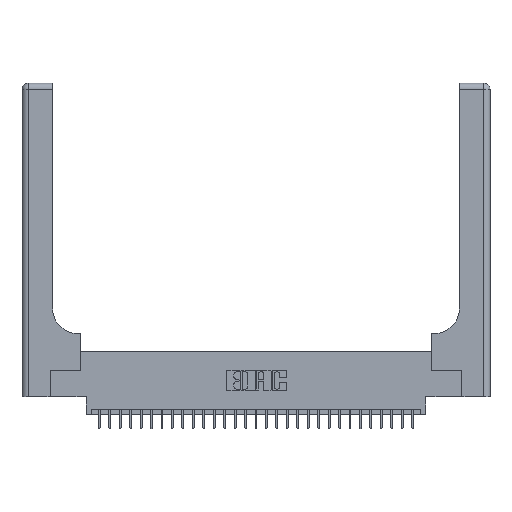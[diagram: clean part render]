
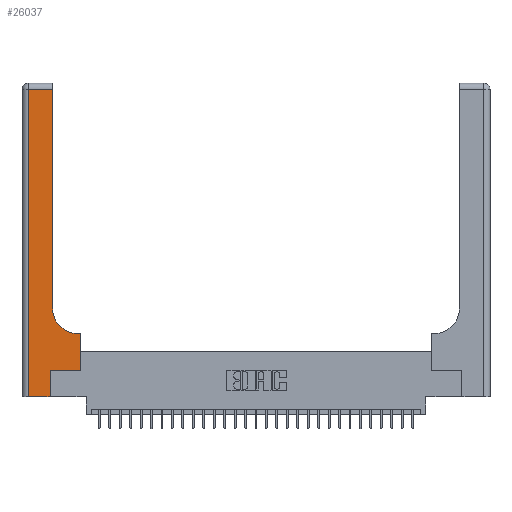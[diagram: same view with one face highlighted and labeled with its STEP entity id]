
A CAD part, top view. The second image highlights one B-rep face of the part: STEP entity #26037.
In plain terms, the highlighted planar face has unit normal (0, 0, 1).
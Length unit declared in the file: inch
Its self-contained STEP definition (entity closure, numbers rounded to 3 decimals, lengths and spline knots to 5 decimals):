
#195 = VERTEX_POINT ( 'NONE', #14794 ) ;
#244 = CARTESIAN_POINT ( 'NONE',  ( 0.269, 0.25, 0.37 ) ) ;
#361 = VERTEX_POINT ( 'NONE', #28563 ) ;
#464 = EDGE_CURVE ( 'NONE', #22327, #3278, #12066, .T. ) ;
#684 = VECTOR ( 'NONE', #4073, 39.37008 ) ;
#1959 = DIRECTION ( 'NONE',  ( 0., 1., 0. ) ) ;
#2272 = DIRECTION ( 'NONE',  ( 1., 0., 0. ) ) ;
#3278 = VERTEX_POINT ( 'NONE', #22702 ) ;
#3656 = VECTOR ( 'NONE', #21701, 39.37008 ) ;
#3835 = ORIENTED_EDGE ( 'NONE', *, *, #9281, .T. ) ;
#4064 = VECTOR ( 'NONE', #29614, 39.37008 ) ;
#4073 = DIRECTION ( 'NONE',  ( 0., 1., 0. ) ) ;
#4226 = ORIENTED_EDGE ( 'NONE', *, *, #27079, .T. ) ;
#4498 = CARTESIAN_POINT ( 'NONE',  ( 0.06, 0., 0.37 ) ) ;
#4769 = VECTOR ( 'NONE', #8406, 39.37008 ) ;
#5786 = EDGE_LOOP ( 'NONE', ( #19864, #14681, #4226, #9943, #3835, #30899, #21212, #20542, #25136 ) ) ;
#5878 = CARTESIAN_POINT ( 'NONE',  ( 0.2915, 0.6, 0.37 ) ) ;
#5907 = CARTESIAN_POINT ( 'NONE',  ( 0., 3., 0.37 ) ) ;
#6124 = CARTESIAN_POINT ( 'NONE',  ( 0.269, 0., 0.37 ) ) ;
#6698 = LINE ( 'NONE', #26444, #17691 ) ;
#7219 = VECTOR ( 'NONE', #29637, 39.37008 ) ;
#7582 = VERTEX_POINT ( 'NONE', #4498 ) ;
#8406 = DIRECTION ( 'NONE',  ( -1., 0., 0. ) ) ;
#8525 = EDGE_CURVE ( 'NONE', #7582, #28544, #30625, .T. ) ;
#9281 = EDGE_CURVE ( 'NONE', #28544, #18430, #23164, .T. ) ;
#9704 = DIRECTION ( 'NONE',  ( 0., 0., -1. ) ) ;
#9731 = CARTESIAN_POINT ( 'NONE',  ( 0.5415, 0.6, 0.37 ) ) ;
#9943 = ORIENTED_EDGE ( 'NONE', *, *, #8525, .T. ) ;
#10630 = FACE_OUTER_BOUND ( 'NONE', #5786, .T. ) ;
#10960 = EDGE_CURVE ( 'NONE', #361, #22327, #27545, .T. ) ;
#11475 = LINE ( 'NONE', #13528, #684 ) ;
#12066 = CIRCLE ( 'NONE', #29768, 0.25 ) ;
#12208 = CARTESIAN_POINT ( 'NONE',  ( 0., 0., 0.37 ) ) ;
#13528 = CARTESIAN_POINT ( 'NONE',  ( 0.5585, 0.25, 0.37 ) ) ;
#14498 = VERTEX_POINT ( 'NONE', #28089 ) ;
#14681 = ORIENTED_EDGE ( 'NONE', *, *, #22768, .T. ) ;
#14794 = CARTESIAN_POINT ( 'NONE',  ( 0.06, 2.94, 0.37 ) ) ;
#15208 = DIRECTION ( 'NONE',  ( -1., 0., 0. ) ) ;
#15681 = CARTESIAN_POINT ( 'NONE',  ( 0.06, 3., 0.37 ) ) ;
#15711 = AXIS2_PLACEMENT_3D ( 'NONE', #5907, #20277, #15208 ) ;
#16486 = DIRECTION ( 'NONE',  ( 1., 0., 0. ) ) ;
#16815 = CARTESIAN_POINT ( 'NONE',  ( 0.5415, 0.85, 0.37 ) ) ;
#17691 = VECTOR ( 'NONE', #1959, 39.37008 ) ;
#17729 = CARTESIAN_POINT ( 'NONE',  ( 0., 2.94, 0.37 ) ) ;
#17749 = LINE ( 'NONE', #15681, #7219 ) ;
#18308 = VECTOR ( 'NONE', #30481, 39.37008 ) ;
#18430 = VERTEX_POINT ( 'NONE', #244 ) ;
#18715 = CARTESIAN_POINT ( 'NONE',  ( 0.269, 0., 0.37 ) ) ;
#19864 = ORIENTED_EDGE ( 'NONE', *, *, #22677, .T. ) ;
#20277 = DIRECTION ( 'NONE',  ( 0., 0., -1. ) ) ;
#20542 = ORIENTED_EDGE ( 'NONE', *, *, #10960, .T. ) ;
#21212 = ORIENTED_EDGE ( 'NONE', *, *, #26813, .T. ) ;
#21546 = CARTESIAN_POINT ( 'NONE',  ( 0.269, 0.25, 0.37 ) ) ;
#21701 = DIRECTION ( 'NONE',  ( 1., 0., 0. ) ) ;
#22327 = VERTEX_POINT ( 'NONE', #9731 ) ;
#22677 = EDGE_CURVE ( 'NONE', #3278, #23268, #6698, .T. ) ;
#22702 = CARTESIAN_POINT ( 'NONE',  ( 0.2915, 0.85, 0.37 ) ) ;
#22768 = EDGE_CURVE ( 'NONE', #23268, #195, #24375, .T. ) ;
#23164 = LINE ( 'NONE', #6124, #18308 ) ;
#23165 = CARTESIAN_POINT ( 'NONE',  ( 0.2915, 2.94, 0.37 ) ) ;
#23268 = VERTEX_POINT ( 'NONE', #23165 ) ;
#24375 = LINE ( 'NONE', #17729, #4064 ) ;
#25136 = ORIENTED_EDGE ( 'NONE', *, *, #464, .T. ) ;
#26037 = ADVANCED_FACE ( 'NONE', ( #10630 ), #27258, .F. ) ;
#26444 = CARTESIAN_POINT ( 'NONE',  ( 0.2915, 3., 0.37 ) ) ;
#26813 = EDGE_CURVE ( 'NONE', #14498, #361, #11475, .T. ) ;
#27079 = EDGE_CURVE ( 'NONE', #195, #7582, #17749, .T. ) ;
#27258 = PLANE ( 'NONE',  #15711 ) ;
#27545 = LINE ( 'NONE', #5878, #4769 ) ;
#28089 = CARTESIAN_POINT ( 'NONE',  ( 0.5585, 0.25, 0.37 ) ) ;
#28544 = VERTEX_POINT ( 'NONE', #18715 ) ;
#28563 = CARTESIAN_POINT ( 'NONE',  ( 0.5585, 0.6, 0.37 ) ) ;
#28679 = LINE ( 'NONE', #21546, #29535 ) ;
#29535 = VECTOR ( 'NONE', #2272, 39.37008 ) ;
#29614 = DIRECTION ( 'NONE',  ( -1., 0., 0. ) ) ;
#29637 = DIRECTION ( 'NONE',  ( 0., -1., 0. ) ) ;
#29768 = AXIS2_PLACEMENT_3D ( 'NONE', #16815, #9704, #16486 ) ;
#29877 = EDGE_CURVE ( 'NONE', #18430, #14498, #28679, .T. ) ;
#30481 = DIRECTION ( 'NONE',  ( 0., 1., 0. ) ) ;
#30625 = LINE ( 'NONE', #12208, #3656 ) ;
#30899 = ORIENTED_EDGE ( 'NONE', *, *, #29877, .T. ) ;
